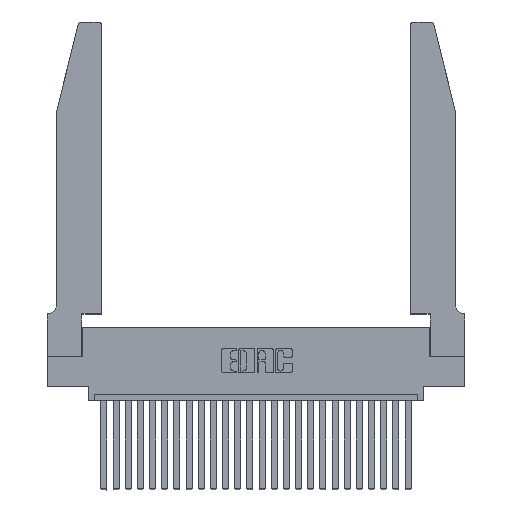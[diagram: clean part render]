
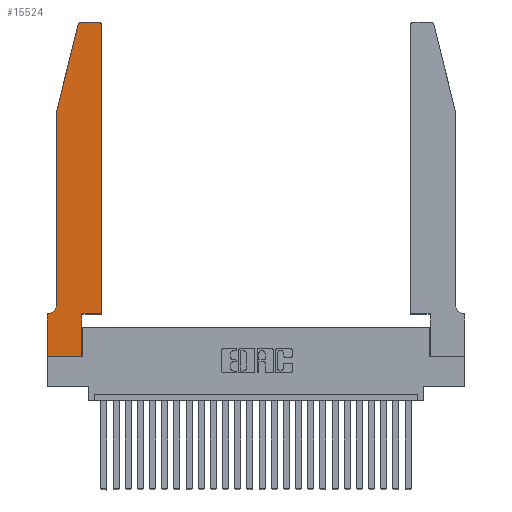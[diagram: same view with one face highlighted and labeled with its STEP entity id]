
A CAD part, top view. The second image highlights one B-rep face of the part: STEP entity #15524.
In plain terms, the highlighted planar face has unit normal (0, 0, 1).
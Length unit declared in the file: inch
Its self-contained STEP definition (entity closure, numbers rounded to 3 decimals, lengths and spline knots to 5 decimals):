
#293 = VECTOR ( 'NONE', #26158, 39.37008 ) ;
#654 = ORIENTED_EDGE ( 'NONE', *, *, #11181, .T. ) ;
#1673 = DIRECTION ( 'NONE',  ( 0., -1., 0. ) ) ;
#2189 = EDGE_CURVE ( 'NONE', #15964, #12653, #21571, .T. ) ;
#2698 = CARTESIAN_POINT ( 'NONE',  ( 0.0755, 2., 0.37 ) ) ;
#2712 = DIRECTION ( 'NONE',  ( 0., 0., 1. ) ) ;
#2866 = AXIS2_PLACEMENT_3D ( 'NONE', #25073, #2712, #20921 ) ;
#3218 = LINE ( 'NONE', #20707, #3522 ) ;
#3342 = VECTOR ( 'NONE', #16851, 39.37008 ) ;
#3388 = CARTESIAN_POINT ( 'NONE',  ( 0.4505, 0.35, 0.37 ) ) ;
#3522 = VECTOR ( 'NONE', #24667, 39.37008 ) ;
#3848 = AXIS2_PLACEMENT_3D ( 'NONE', #16485, #20588, #12624 ) ;
#3899 = CIRCLE ( 'NONE', #3848, 0.03 ) ;
#4201 = VERTEX_POINT ( 'NONE', #7649 ) ;
#4429 = EDGE_CURVE ( 'NONE', #4201, #12137, #6116, .T. ) ;
#4888 = ORIENTED_EDGE ( 'NONE', *, *, #24524, .T. ) ;
#5387 = AXIS2_PLACEMENT_3D ( 'NONE', #10062, #16226, #8346 ) ;
#5443 = ORIENTED_EDGE ( 'NONE', *, *, #4429, .T. ) ;
#5573 = CARTESIAN_POINT ( 'NONE',  ( 0., 0.35, 0.37 ) ) ;
#5933 = EDGE_CURVE ( 'NONE', #18274, #26044, #15966, .T. ) ;
#6116 = LINE ( 'NONE', #3388, #24620 ) ;
#6198 = ORIENTED_EDGE ( 'NONE', *, *, #24070, .T. ) ;
#6973 = CARTESIAN_POINT ( 'NONE',  ( 0., 0., 0.37 ) ) ;
#7530 = DIRECTION ( 'NONE',  ( -1., 0., 0. ) ) ;
#7649 = CARTESIAN_POINT ( 'NONE',  ( 0.2865, 0.35, 0.37 ) ) ;
#8119 = DIRECTION ( 'NONE',  ( -0.239, -0.971, 0. ) ) ;
#8282 = LINE ( 'NONE', #10178, #26451 ) ;
#8346 = DIRECTION ( 'NONE',  ( -1., 0., 0. ) ) ;
#8440 = CARTESIAN_POINT ( 'NONE',  ( 0.25487, 2.72718, 0.37 ) ) ;
#8457 = VERTEX_POINT ( 'NONE', #14404 ) ;
#8861 = CARTESIAN_POINT ( 'NONE',  ( 0.284, 2.75, 0.37 ) ) ;
#9065 = VERTEX_POINT ( 'NONE', #11859 ) ;
#9191 = EDGE_CURVE ( 'NONE', #22029, #10046, #3218, .T. ) ;
#9310 = CIRCLE ( 'NONE', #5387, 0.07 ) ;
#10046 = VERTEX_POINT ( 'NONE', #8861 ) ;
#10062 = CARTESIAN_POINT ( 'NONE',  ( 0.0055, 0.42, 0.37 ) ) ;
#10178 = CARTESIAN_POINT ( 'NONE',  ( 0.0755, 2., 0.37 ) ) ;
#10750 = EDGE_CURVE ( 'NONE', #26044, #15964, #13662, .T. ) ;
#10871 = AXIS2_PLACEMENT_3D ( 'NONE', #5573, #26150, #15946 ) ;
#11163 = ORIENTED_EDGE ( 'NONE', *, *, #5933, .T. ) ;
#11181 = EDGE_CURVE ( 'NONE', #14668, #9065, #24160, .T. ) ;
#11847 = CIRCLE ( 'NONE', #2866, 0.03 ) ;
#11859 = CARTESIAN_POINT ( 'NONE',  ( 0.0755, 0.42, 0.37 ) ) ;
#11926 = CARTESIAN_POINT ( 'NONE',  ( 0.4505, 0.35, 0.37 ) ) ;
#12137 = VERTEX_POINT ( 'NONE', #15512 ) ;
#12446 = VECTOR ( 'NONE', #7530, 39.37008 ) ;
#12574 = DIRECTION ( 'NONE',  ( 1., 0., 0. ) ) ;
#12624 = DIRECTION ( 'NONE',  ( 1., 0., 0. ) ) ;
#12653 = VERTEX_POINT ( 'NONE', #19186 ) ;
#12849 = CARTESIAN_POINT ( 'NONE',  ( 0., 0.35, 0.37 ) ) ;
#13585 = DIRECTION ( 'NONE',  ( 1., 0., 0. ) ) ;
#13662 = LINE ( 'NONE', #24249, #21009 ) ;
#14107 = DIRECTION ( 'NONE',  ( 0., -1., 0. ) ) ;
#14404 = CARTESIAN_POINT ( 'NONE',  ( 0.4505, 2.72, 0.37 ) ) ;
#14668 = VERTEX_POINT ( 'NONE', #2698 ) ;
#14697 = CARTESIAN_POINT ( 'NONE',  ( 0.2865, 0.35, 0.37 ) ) ;
#15222 = EDGE_LOOP ( 'NONE', ( #23203, #20323, #6198, #654, #25960, #11163, #21113, #16542, #20383, #5443, #4888, #19431 ) ) ;
#15498 = VECTOR ( 'NONE', #12574, 39.37008 ) ;
#15512 = CARTESIAN_POINT ( 'NONE',  ( 0.4505, 0.35, 0.37 ) ) ;
#15524 = ADVANCED_FACE ( 'NONE', ( #19529 ), #19971, .T. ) ;
#15676 = EDGE_CURVE ( 'NONE', #9065, #18274, #9310, .T. ) ;
#15694 = CARTESIAN_POINT ( 'NONE',  ( 0.0755, 0.35, 0.37 ) ) ;
#15890 = EDGE_CURVE ( 'NONE', #10046, #22676, #11847, .T. ) ;
#15946 = DIRECTION ( 'NONE',  ( 1., 0., 0. ) ) ;
#15964 = VERTEX_POINT ( 'NONE', #6973 ) ;
#15966 = LINE ( 'NONE', #15694, #12446 ) ;
#16097 = CARTESIAN_POINT ( 'NONE',  ( 0.0055, 0.35, 0.37 ) ) ;
#16226 = DIRECTION ( 'NONE',  ( 0., 0., -1. ) ) ;
#16478 = LINE ( 'NONE', #14697, #3342 ) ;
#16485 = CARTESIAN_POINT ( 'NONE',  ( 0.4205, 2.72, 0.37 ) ) ;
#16542 = ORIENTED_EDGE ( 'NONE', *, *, #2189, .T. ) ;
#16851 = DIRECTION ( 'NONE',  ( 0., 1., 0. ) ) ;
#18274 = VERTEX_POINT ( 'NONE', #16097 ) ;
#18625 = EDGE_CURVE ( 'NONE', #12653, #4201, #16478, .T. ) ;
#19186 = CARTESIAN_POINT ( 'NONE',  ( 0.2865, 0., 0.37 ) ) ;
#19431 = ORIENTED_EDGE ( 'NONE', *, *, #26391, .T. ) ;
#19529 = FACE_OUTER_BOUND ( 'NONE', #15222, .T. ) ;
#19971 = PLANE ( 'NONE',  #10871 ) ;
#20323 = ORIENTED_EDGE ( 'NONE', *, *, #15890, .T. ) ;
#20383 = ORIENTED_EDGE ( 'NONE', *, *, #18625, .T. ) ;
#20588 = DIRECTION ( 'NONE',  ( 0., 0., 1. ) ) ;
#20707 = CARTESIAN_POINT ( 'NONE',  ( 0.2605, 2.75, 0.37 ) ) ;
#20741 = LINE ( 'NONE', #11926, #293 ) ;
#20785 = CARTESIAN_POINT ( 'NONE',  ( 0., 0., 0.37 ) ) ;
#20921 = DIRECTION ( 'NONE',  ( 1., 0., 0. ) ) ;
#21009 = VECTOR ( 'NONE', #14107, 39.37008 ) ;
#21113 = ORIENTED_EDGE ( 'NONE', *, *, #10750, .T. ) ;
#21571 = LINE ( 'NONE', #20785, #15498 ) ;
#22029 = VERTEX_POINT ( 'NONE', #22931 ) ;
#22676 = VERTEX_POINT ( 'NONE', #8440 ) ;
#22931 = CARTESIAN_POINT ( 'NONE',  ( 0.4205, 2.75, 0.37 ) ) ;
#23203 = ORIENTED_EDGE ( 'NONE', *, *, #9191, .T. ) ;
#23524 = VECTOR ( 'NONE', #1673, 39.37008 ) ;
#24070 = EDGE_CURVE ( 'NONE', #22676, #14668, #8282, .T. ) ;
#24160 = LINE ( 'NONE', #26020, #23524 ) ;
#24249 = CARTESIAN_POINT ( 'NONE',  ( 0., 0., 0.37 ) ) ;
#24524 = EDGE_CURVE ( 'NONE', #12137, #8457, #20741, .T. ) ;
#24620 = VECTOR ( 'NONE', #13585, 39.37008 ) ;
#24667 = DIRECTION ( 'NONE',  ( -1., 0., 0. ) ) ;
#25073 = CARTESIAN_POINT ( 'NONE',  ( 0.284, 2.72, 0.37 ) ) ;
#25960 = ORIENTED_EDGE ( 'NONE', *, *, #15676, .T. ) ;
#26020 = CARTESIAN_POINT ( 'NONE',  ( 0.0755, 2., 0.37 ) ) ;
#26044 = VERTEX_POINT ( 'NONE', #12849 ) ;
#26150 = DIRECTION ( 'NONE',  ( 0., 0., 1. ) ) ;
#26158 = DIRECTION ( 'NONE',  ( 0., 1., 0. ) ) ;
#26391 = EDGE_CURVE ( 'NONE', #8457, #22029, #3899, .T. ) ;
#26451 = VECTOR ( 'NONE', #8119, 39.37008 ) ;
